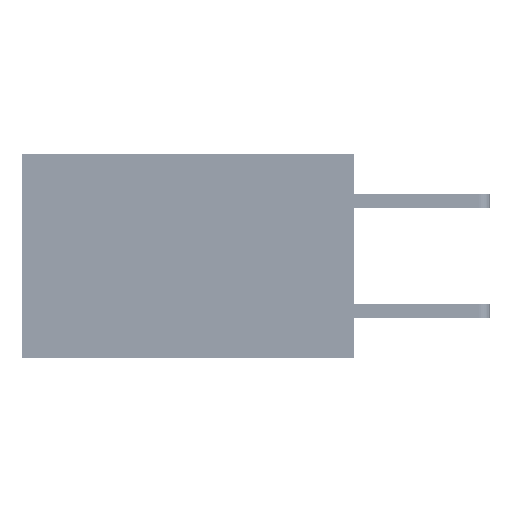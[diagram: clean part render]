
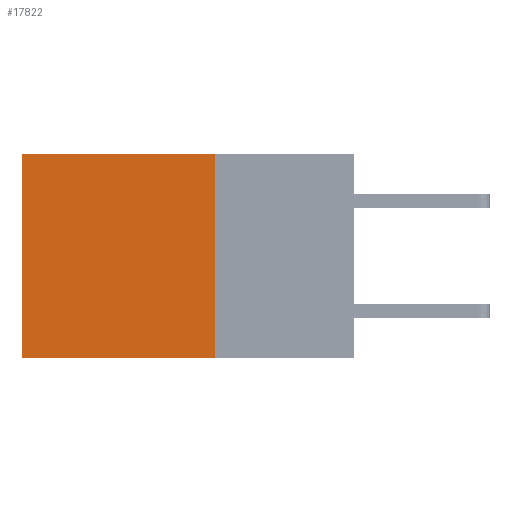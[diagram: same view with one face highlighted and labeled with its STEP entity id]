
A CAD part, left-side view. The second image highlights one B-rep face of the part: STEP entity #17822.
In plain terms, the highlighted planar face has unit normal (-1, 0, 0).
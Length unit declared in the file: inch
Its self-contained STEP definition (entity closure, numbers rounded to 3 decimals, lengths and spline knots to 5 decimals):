
#91 = LINE ( 'NONE', #43919, #10943 ) ;
#2001 = DIRECTION ( 'NONE',  ( 0., 0., -1. ) ) ;
#3755 = CARTESIAN_POINT ( 'NONE',  ( 0.2875, 0.25, -0.37 ) ) ;
#4762 = EDGE_CURVE ( 'NONE', #5310, #44409, #40307, .T. ) ;
#4955 = ORIENTED_EDGE ( 'NONE', *, *, #43964, .T. ) ;
#5310 = VERTEX_POINT ( 'NONE', #3755 ) ;
#7446 = AXIS2_PLACEMENT_3D ( 'NONE', #17463, #33197, #2001 ) ;
#10943 = VECTOR ( 'NONE', #24302, 39.37008 ) ;
#17463 = CARTESIAN_POINT ( 'NONE',  ( 0.2875, 0.25, 0. ) ) ;
#17617 = VECTOR ( 'NONE', #23844, 39.37008 ) ;
#17822 = ADVANCED_FACE ( 'NONE', ( #25466 ), #48396, .F. ) ;
#19442 = VECTOR ( 'NONE', #40550, 39.37008 ) ;
#19561 = ORIENTED_EDGE ( 'NONE', *, *, #35189, .T. ) ;
#19790 = CARTESIAN_POINT ( 'NONE',  ( 0.2875, 0.6, 0. ) ) ;
#20725 = CARTESIAN_POINT ( 'NONE',  ( 0.2875, 0.25, -0.37 ) ) ;
#22863 = CARTESIAN_POINT ( 'NONE',  ( 0.2875, 0.6, -0.37 ) ) ;
#23844 = DIRECTION ( 'NONE',  ( 0., 1., 0. ) ) ;
#24302 = DIRECTION ( 'NONE',  ( 0., 1., 0. ) ) ;
#25466 = FACE_OUTER_BOUND ( 'NONE', #50428, .T. ) ;
#26117 = CARTESIAN_POINT ( 'NONE',  ( 0.2875, 0.6, 0. ) ) ;
#26636 = EDGE_CURVE ( 'NONE', #33385, #5310, #37470, .T. ) ;
#26786 = DIRECTION ( 'NONE',  ( 0., 0., -1. ) ) ;
#28563 = VECTOR ( 'NONE', #26786, 39.37008 ) ;
#30109 = CARTESIAN_POINT ( 'NONE',  ( 0.2875, 0.25, 0. ) ) ;
#33197 = DIRECTION ( 'NONE',  ( 1., 0., 0. ) ) ;
#33385 = VERTEX_POINT ( 'NONE', #30109 ) ;
#33631 = ORIENTED_EDGE ( 'NONE', *, *, #26636, .F. ) ;
#35189 = EDGE_CURVE ( 'NONE', #33385, #46521, #91, .T. ) ;
#37470 = LINE ( 'NONE', #49321, #19442 ) ;
#40307 = LINE ( 'NONE', #20725, #17617 ) ;
#40550 = DIRECTION ( 'NONE',  ( 0., 0., -1. ) ) ;
#43919 = CARTESIAN_POINT ( 'NONE',  ( 0.2875, 0.25, 0. ) ) ;
#43964 = EDGE_CURVE ( 'NONE', #46521, #44409, #47638, .T. ) ;
#44409 = VERTEX_POINT ( 'NONE', #22863 ) ;
#46521 = VERTEX_POINT ( 'NONE', #26117 ) ;
#47638 = LINE ( 'NONE', #19790, #28563 ) ;
#48396 = PLANE ( 'NONE',  #7446 ) ;
#49321 = CARTESIAN_POINT ( 'NONE',  ( 0.2875, 0.25, 0. ) ) ;
#49704 = ORIENTED_EDGE ( 'NONE', *, *, #4762, .F. ) ;
#50428 = EDGE_LOOP ( 'NONE', ( #4955, #49704, #33631, #19561 ) ) ;
